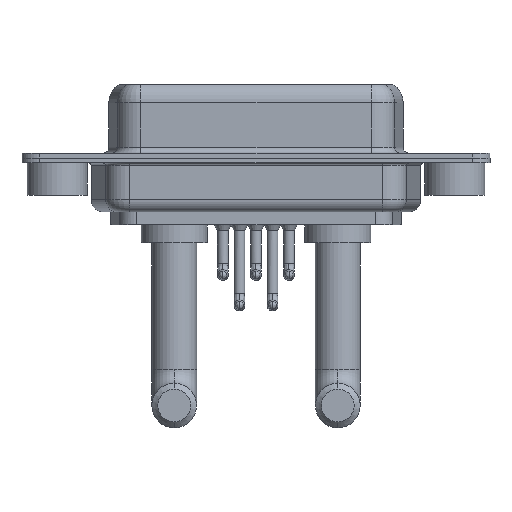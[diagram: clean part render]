
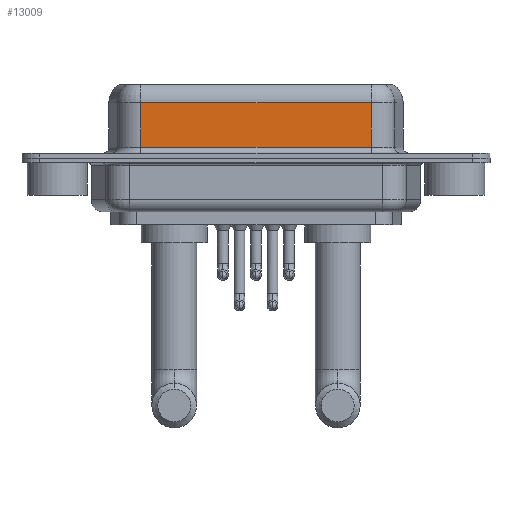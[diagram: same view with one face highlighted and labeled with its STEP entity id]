
A CAD part, front view. The second image highlights one B-rep face of the part: STEP entity #13009.
In plain terms, the highlighted planar face has unit normal (0, -1, 0).
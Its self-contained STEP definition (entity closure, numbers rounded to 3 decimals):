
#227 = EDGE_CURVE ( 'NONE', #5398, #16799, #8766, .T. ) ;
#278 = VECTOR ( 'NONE', #14914, 1000. ) ;
#303 = FACE_OUTER_BOUND ( 'NONE', #16386, .T. ) ;
#2424 = VERTEX_POINT ( 'NONE', #5447 ) ;
#2501 = LINE ( 'NONE', #12839, #13954 ) ;
#4243 = LINE ( 'NONE', #14606, #13434 ) ;
#5171 = AXIS2_PLACEMENT_3D ( 'NONE', #7973, #10593, #13130 ) ;
#5310 = EDGE_CURVE ( 'NONE', #2424, #16799, #2501, .T. ) ;
#5398 = VERTEX_POINT ( 'NONE', #12810 ) ;
#5447 = CARTESIAN_POINT ( 'NONE',  ( 26.287, -3.95, 4.65 ) ) ;
#6357 = CARTESIAN_POINT ( 'NONE',  ( 26.287, -3.95, 0.9 ) ) ;
#6975 = EDGE_CURVE ( 'NONE', #16364, #5398, #4243, .T. ) ;
#7566 = ORIENTED_EDGE ( 'NONE', *, *, #227, .T. ) ;
#7973 = CARTESIAN_POINT ( 'NONE',  ( 26.287, -3.95, 6.4 ) ) ;
#8231 = PLANE ( 'NONE',  #5171 ) ;
#8766 = LINE ( 'NONE', #6357, #10759 ) ;
#9069 = DIRECTION ( 'NONE',  ( 0., 0., -1. ) ) ;
#10593 = DIRECTION ( 'NONE',  ( 0., 1., 0. ) ) ;
#10759 = VECTOR ( 'NONE', #12716, 1000. ) ;
#12020 = ORIENTED_EDGE ( 'NONE', *, *, #5310, .F. ) ;
#12174 = CARTESIAN_POINT ( 'NONE',  ( 26.287, -3.95, 4.65 ) ) ;
#12716 = DIRECTION ( 'NONE',  ( 1., 0., 0. ) ) ;
#12810 = CARTESIAN_POINT ( 'NONE',  ( 7.013, -3.95, 0.9 ) ) ;
#12839 = CARTESIAN_POINT ( 'NONE',  ( 26.287, -3.95, 6.4 ) ) ;
#13009 = ADVANCED_FACE ( 'NONE', ( #303 ), #8231, .F. ) ;
#13130 = DIRECTION ( 'NONE',  ( 0., 0., 1. ) ) ;
#13434 = VECTOR ( 'NONE', #14201, 1000. ) ;
#13645 = ORIENTED_EDGE ( 'NONE', *, *, #14867, .T. ) ;
#13954 = VECTOR ( 'NONE', #9069, 1000. ) ;
#14201 = DIRECTION ( 'NONE',  ( 0., 0., -1. ) ) ;
#14606 = CARTESIAN_POINT ( 'NONE',  ( 7.013, -3.95, 6.4 ) ) ;
#14746 = CARTESIAN_POINT ( 'NONE',  ( 7.013, -3.95, 4.65 ) ) ;
#14867 = EDGE_CURVE ( 'NONE', #2424, #16364, #16281, .T. ) ;
#14914 = DIRECTION ( 'NONE',  ( -1., 0., 0. ) ) ;
#15401 = CARTESIAN_POINT ( 'NONE',  ( 26.287, -3.95, 0.9 ) ) ;
#15917 = ORIENTED_EDGE ( 'NONE', *, *, #6975, .T. ) ;
#16281 = LINE ( 'NONE', #12174, #278 ) ;
#16364 = VERTEX_POINT ( 'NONE', #14746 ) ;
#16386 = EDGE_LOOP ( 'NONE', ( #12020, #13645, #15917, #7566 ) ) ;
#16799 = VERTEX_POINT ( 'NONE', #15401 ) ;
